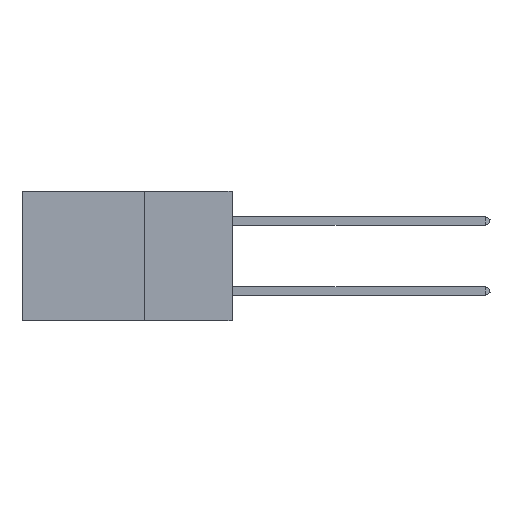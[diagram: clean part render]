
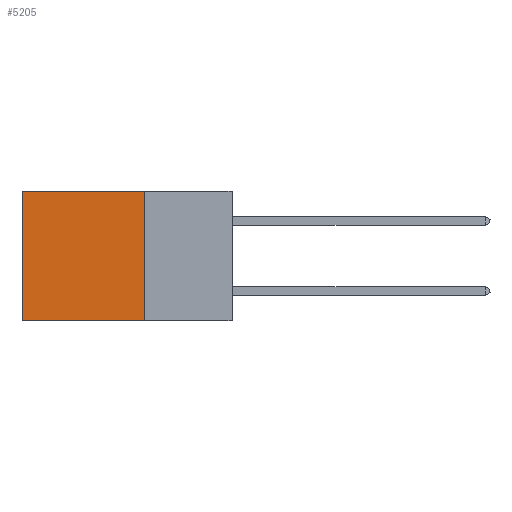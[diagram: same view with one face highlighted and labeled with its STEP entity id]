
A CAD part, left-side view. The second image highlights one B-rep face of the part: STEP entity #5205.
In plain terms, the highlighted planar face has unit normal (-1, 0, 0).
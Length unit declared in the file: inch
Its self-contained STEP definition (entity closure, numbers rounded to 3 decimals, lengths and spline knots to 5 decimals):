
#539 = FACE_OUTER_BOUND ( 'NONE', #38503, .T. ) ;
#616 = CARTESIAN_POINT ( 'NONE',  ( 0.2875, 0.25, 0. ) ) ;
#895 = DIRECTION ( 'NONE',  ( 0., 1., 0. ) ) ;
#2045 = AXIS2_PLACEMENT_3D ( 'NONE', #30479, #34000, #26332 ) ;
#3423 = LINE ( 'NONE', #27658, #45501 ) ;
#4595 = DIRECTION ( 'NONE',  ( 0., 0., -1. ) ) ;
#5149 = PLANE ( 'NONE',  #2045 ) ;
#5205 = ADVANCED_FACE ( 'NONE', ( #539 ), #5149, .F. ) ;
#6239 = CARTESIAN_POINT ( 'NONE',  ( 0.2875, 0.6, 0. ) ) ;
#6889 = VERTEX_POINT ( 'NONE', #32306 ) ;
#14186 = EDGE_CURVE ( 'NONE', #16570, #42111, #24011, .T. ) ;
#16570 = VERTEX_POINT ( 'NONE', #43185 ) ;
#17475 = VECTOR ( 'NONE', #4595, 39.37008 ) ;
#23584 = ORIENTED_EDGE ( 'NONE', *, *, #29925, .T. ) ;
#24011 = LINE ( 'NONE', #34363, #26293 ) ;
#25620 = DIRECTION ( 'NONE',  ( 0., 0., -1. ) ) ;
#26293 = VECTOR ( 'NONE', #895, 39.37008 ) ;
#26332 = DIRECTION ( 'NONE',  ( 0., 0., -1. ) ) ;
#26962 = ORIENTED_EDGE ( 'NONE', *, *, #14186, .T. ) ;
#27658 = CARTESIAN_POINT ( 'NONE',  ( 0.2875, 0.25, -0.37 ) ) ;
#28754 = VECTOR ( 'NONE', #25620, 39.37008 ) ;
#29162 = CARTESIAN_POINT ( 'NONE',  ( 0.2875, 0.6, -0.37 ) ) ;
#29925 = EDGE_CURVE ( 'NONE', #42111, #33476, #45173, .T. ) ;
#30479 = CARTESIAN_POINT ( 'NONE',  ( 0.2875, 0.25, 0. ) ) ;
#32302 = EDGE_CURVE ( 'NONE', #6889, #33476, #3423, .T. ) ;
#32306 = CARTESIAN_POINT ( 'NONE',  ( 0.2875, 0.25, -0.37 ) ) ;
#33476 = VERTEX_POINT ( 'NONE', #29162 ) ;
#34000 = DIRECTION ( 'NONE',  ( 1., 0., 0. ) ) ;
#34363 = CARTESIAN_POINT ( 'NONE',  ( 0.2875, 0.25, 0. ) ) ;
#35142 = ORIENTED_EDGE ( 'NONE', *, *, #32302, .F. ) ;
#38304 = EDGE_CURVE ( 'NONE', #16570, #6889, #42478, .T. ) ;
#38503 = EDGE_LOOP ( 'NONE', ( #23584, #35142, #42829, #26962 ) ) ;
#40081 = CARTESIAN_POINT ( 'NONE',  ( 0.2875, 0.6, 0. ) ) ;
#41937 = DIRECTION ( 'NONE',  ( 0., 1., 0. ) ) ;
#42111 = VERTEX_POINT ( 'NONE', #6239 ) ;
#42478 = LINE ( 'NONE', #616, #17475 ) ;
#42829 = ORIENTED_EDGE ( 'NONE', *, *, #38304, .F. ) ;
#43185 = CARTESIAN_POINT ( 'NONE',  ( 0.2875, 0.25, 0. ) ) ;
#45173 = LINE ( 'NONE', #40081, #28754 ) ;
#45501 = VECTOR ( 'NONE', #41937, 39.37008 ) ;
